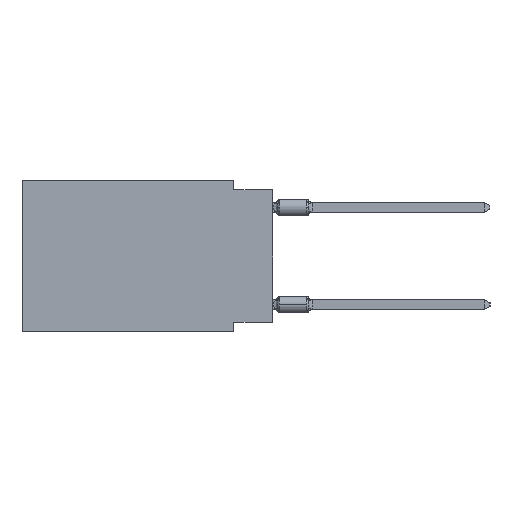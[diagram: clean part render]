
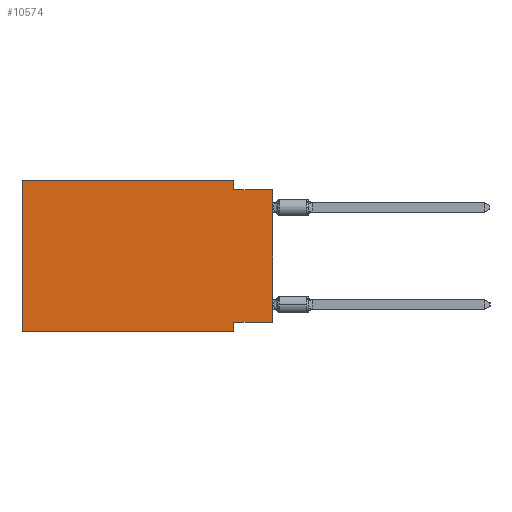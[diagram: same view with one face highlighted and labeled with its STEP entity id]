
A CAD part, left-side view. The second image highlights one B-rep face of the part: STEP entity #10574.
In plain terms, the highlighted planar face has unit normal (-1, 0, 0).
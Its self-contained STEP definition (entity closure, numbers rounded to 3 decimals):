
#155 = DIRECTION ( 'NONE',  ( 0., 0., 1. ) ) ;
#2052 = DIRECTION ( 'NONE',  ( 0., -1., 0. ) ) ;
#2768 = VECTOR ( 'NONE', #155, 1000. ) ;
#2786 = EDGE_LOOP ( 'NONE', ( #18124, #21940, #21843, #27514, #21755, #13036, #7659, #21054 ) ) ;
#3077 = CARTESIAN_POINT ( 'NONE',  ( 0., 16.383, 0. ) ) ;
#3473 = DIRECTION ( 'NONE',  ( 1., 0., 0. ) ) ;
#3975 = EDGE_CURVE ( 'NONE', #17008, #27835, #26654, .T. ) ;
#4206 = DIRECTION ( 'NONE',  ( 0., 0., -1. ) ) ;
#7400 = DIRECTION ( 'NONE',  ( 0., -1., 0. ) ) ;
#7478 = VERTEX_POINT ( 'NONE', #29766 ) ;
#7497 = CARTESIAN_POINT ( 'NONE',  ( 0., 16.383, -9.906 ) ) ;
#7541 = VERTEX_POINT ( 'NONE', #23128 ) ;
#7659 = ORIENTED_EDGE ( 'NONE', *, *, #11071, .F. ) ;
#7710 = CARTESIAN_POINT ( 'NONE',  ( 0., 2.54, -0.635 ) ) ;
#8047 = DIRECTION ( 'NONE',  ( 0., 0., -1. ) ) ;
#8882 = EDGE_CURVE ( 'NONE', #7541, #19310, #16490, .T. ) ;
#9360 = DIRECTION ( 'NONE',  ( 0., 0., -1. ) ) ;
#9908 = EDGE_CURVE ( 'NONE', #7541, #7478, #24009, .T. ) ;
#10413 = PLANE ( 'NONE',  #25801 ) ;
#10574 = ADVANCED_FACE ( 'NONE', ( #25090 ), #10413, .F. ) ;
#10578 = EDGE_CURVE ( 'NONE', #24055, #19310, #27286, .T. ) ;
#11071 = EDGE_CURVE ( 'NONE', #7478, #27835, #23865, .T. ) ;
#11980 = LINE ( 'NONE', #26667, #2768 ) ;
#12478 = VERTEX_POINT ( 'NONE', #3077 ) ;
#12832 = VERTEX_POINT ( 'NONE', #14729 ) ;
#13036 = ORIENTED_EDGE ( 'NONE', *, *, #3975, .T. ) ;
#13201 = VECTOR ( 'NONE', #29963, 1000. ) ;
#13642 = VECTOR ( 'NONE', #2052, 1000. ) ;
#13661 = EDGE_CURVE ( 'NONE', #12832, #24055, #16197, .T. ) ;
#14729 = CARTESIAN_POINT ( 'NONE',  ( 0., 2.54, 0. ) ) ;
#15302 = CARTESIAN_POINT ( 'NONE',  ( 0., 0., -0.635 ) ) ;
#16044 = CARTESIAN_POINT ( 'NONE',  ( 0., 0., 0. ) ) ;
#16197 = LINE ( 'NONE', #18400, #20950 ) ;
#16490 = LINE ( 'NONE', #16044, #30250 ) ;
#17008 = VERTEX_POINT ( 'NONE', #7497 ) ;
#18124 = ORIENTED_EDGE ( 'NONE', *, *, #8882, .T. ) ;
#18400 = CARTESIAN_POINT ( 'NONE',  ( 0., 2.54, 0. ) ) ;
#18591 = CARTESIAN_POINT ( 'NONE',  ( 0., 2.54, -9.906 ) ) ;
#19310 = VERTEX_POINT ( 'NONE', #26447 ) ;
#20950 = VECTOR ( 'NONE', #4206, 1000. ) ;
#21054 = ORIENTED_EDGE ( 'NONE', *, *, #9908, .F. ) ;
#21755 = ORIENTED_EDGE ( 'NONE', *, *, #26197, .F. ) ;
#21759 = CARTESIAN_POINT ( 'NONE',  ( 0., 16.383, 0. ) ) ;
#21843 = ORIENTED_EDGE ( 'NONE', *, *, #13661, .F. ) ;
#21940 = ORIENTED_EDGE ( 'NONE', *, *, #10578, .F. ) ;
#22269 = VECTOR ( 'NONE', #9360, 1000. ) ;
#23128 = CARTESIAN_POINT ( 'NONE',  ( 0., 0., -9.271 ) ) ;
#23717 = CARTESIAN_POINT ( 'NONE',  ( 0., 2.54, -9.906 ) ) ;
#23865 = LINE ( 'NONE', #23717, #22269 ) ;
#24009 = LINE ( 'NONE', #29365, #29794 ) ;
#24055 = VERTEX_POINT ( 'NONE', #7710 ) ;
#25090 = FACE_OUTER_BOUND ( 'NONE', #2786, .T. ) ;
#25112 = VECTOR ( 'NONE', #7400, 1000. ) ;
#25801 = AXIS2_PLACEMENT_3D ( 'NONE', #29639, #3473, #8047 ) ;
#26035 = CARTESIAN_POINT ( 'NONE',  ( 0., 16.383, -9.906 ) ) ;
#26197 = EDGE_CURVE ( 'NONE', #17008, #12478, #11980, .T. ) ;
#26232 = DIRECTION ( 'NONE',  ( 0., 1., 0. ) ) ;
#26447 = CARTESIAN_POINT ( 'NONE',  ( 0., 0., -0.635 ) ) ;
#26654 = LINE ( 'NONE', #26035, #13642 ) ;
#26667 = CARTESIAN_POINT ( 'NONE',  ( 0., 16.383, 0. ) ) ;
#27117 = LINE ( 'NONE', #21759, #25112 ) ;
#27286 = LINE ( 'NONE', #15302, #13201 ) ;
#27514 = ORIENTED_EDGE ( 'NONE', *, *, #30555, .F. ) ;
#27835 = VERTEX_POINT ( 'NONE', #18591 ) ;
#28022 = DIRECTION ( 'NONE',  ( 0., 0., 1. ) ) ;
#29365 = CARTESIAN_POINT ( 'NONE',  ( 0., 0., -9.271 ) ) ;
#29639 = CARTESIAN_POINT ( 'NONE',  ( 0., 16.383, 0. ) ) ;
#29766 = CARTESIAN_POINT ( 'NONE',  ( 0., 2.54, -9.271 ) ) ;
#29794 = VECTOR ( 'NONE', #26232, 1000. ) ;
#29963 = DIRECTION ( 'NONE',  ( 0., -1., 0. ) ) ;
#30250 = VECTOR ( 'NONE', #28022, 1000. ) ;
#30555 = EDGE_CURVE ( 'NONE', #12478, #12832, #27117, .T. ) ;
